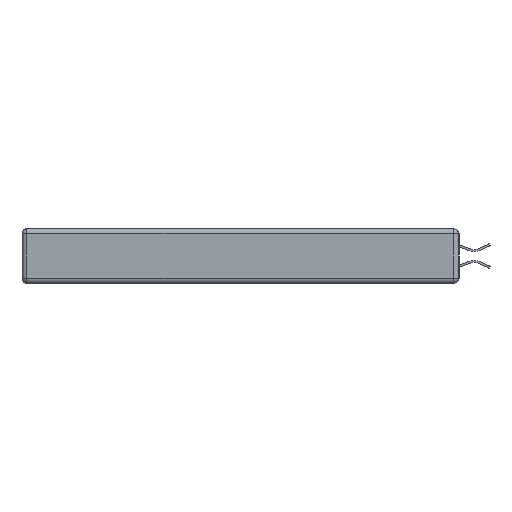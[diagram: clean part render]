
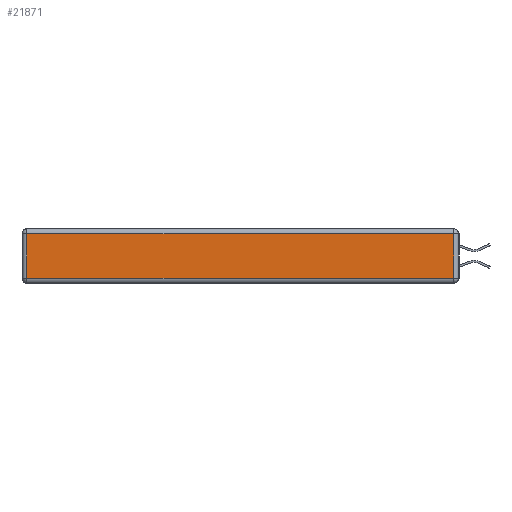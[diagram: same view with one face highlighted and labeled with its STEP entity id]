
A CAD part, left-side view. The second image highlights one B-rep face of the part: STEP entity #21871.
In plain terms, the highlighted planar face has unit normal (-1, 0, 0).
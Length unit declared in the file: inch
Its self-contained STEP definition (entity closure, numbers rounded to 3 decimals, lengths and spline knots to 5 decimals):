
#23 = CARTESIAN_POINT ( 'NONE',  ( 0., 2.72, -0.313 ) ) ;
#171 = ORIENTED_EDGE ( 'NONE', *, *, #14660, .T. ) ;
#1970 = ORIENTED_EDGE ( 'NONE', *, *, #21735, .T. ) ;
#3237 = CARTESIAN_POINT ( 'NONE',  ( 0., 2.75, -0.03 ) ) ;
#4489 = CARTESIAN_POINT ( 'NONE',  ( 0., 0., -0.343 ) ) ;
#5820 = VERTEX_POINT ( 'NONE', #20007 ) ;
#6055 = LINE ( 'NONE', #3237, #23326 ) ;
#8141 = DIRECTION ( 'NONE',  ( -1., 0., 0. ) ) ;
#8203 = DIRECTION ( 'NONE',  ( 0., 0., 1. ) ) ;
#8211 = AXIS2_PLACEMENT_3D ( 'NONE', #4489, #8141, #20809 ) ;
#9545 = DIRECTION ( 'NONE',  ( 0., 0., -1. ) ) ;
#9554 = CARTESIAN_POINT ( 'NONE',  ( 0., 0., -0.313 ) ) ;
#10002 = LINE ( 'NONE', #13740, #19096 ) ;
#10386 = EDGE_LOOP ( 'NONE', ( #1970, #13433, #15164, #171 ) ) ;
#10653 = VECTOR ( 'NONE', #13204, 39.37008 ) ;
#11680 = PLANE ( 'NONE',  #8211 ) ;
#11883 = VECTOR ( 'NONE', #9545, 39.37008 ) ;
#12569 = VERTEX_POINT ( 'NONE', #21474 ) ;
#13204 = DIRECTION ( 'NONE',  ( 0., -1., 0. ) ) ;
#13291 = VERTEX_POINT ( 'NONE', #20029 ) ;
#13433 = ORIENTED_EDGE ( 'NONE', *, *, #19342, .T. ) ;
#13740 = CARTESIAN_POINT ( 'NONE',  ( 0., 0.03, -0.343 ) ) ;
#14660 = EDGE_CURVE ( 'NONE', #5820, #20808, #18152, .T. ) ;
#15164 = ORIENTED_EDGE ( 'NONE', *, *, #19537, .T. ) ;
#17196 = FACE_OUTER_BOUND ( 'NONE', #10386, .T. ) ;
#18027 = LINE ( 'NONE', #9554, #10653 ) ;
#18152 = LINE ( 'NONE', #18671, #11883 ) ;
#18671 = CARTESIAN_POINT ( 'NONE',  ( 0., 2.72, -0.343 ) ) ;
#19096 = VECTOR ( 'NONE', #8203, 39.37008 ) ;
#19342 = EDGE_CURVE ( 'NONE', #12569, #13291, #10002, .T. ) ;
#19537 = EDGE_CURVE ( 'NONE', #13291, #5820, #6055, .T. ) ;
#19597 = DIRECTION ( 'NONE',  ( 0., 1., 0. ) ) ;
#20007 = CARTESIAN_POINT ( 'NONE',  ( 0., 2.72, -0.03 ) ) ;
#20029 = CARTESIAN_POINT ( 'NONE',  ( 0., 0.03, -0.03 ) ) ;
#20808 = VERTEX_POINT ( 'NONE', #23 ) ;
#20809 = DIRECTION ( 'NONE',  ( 0., 0., 1. ) ) ;
#21474 = CARTESIAN_POINT ( 'NONE',  ( 0., 0.03, -0.313 ) ) ;
#21735 = EDGE_CURVE ( 'NONE', #20808, #12569, #18027, .T. ) ;
#21871 = ADVANCED_FACE ( 'NONE', ( #17196 ), #11680, .T. ) ;
#23326 = VECTOR ( 'NONE', #19597, 39.37008 ) ;
